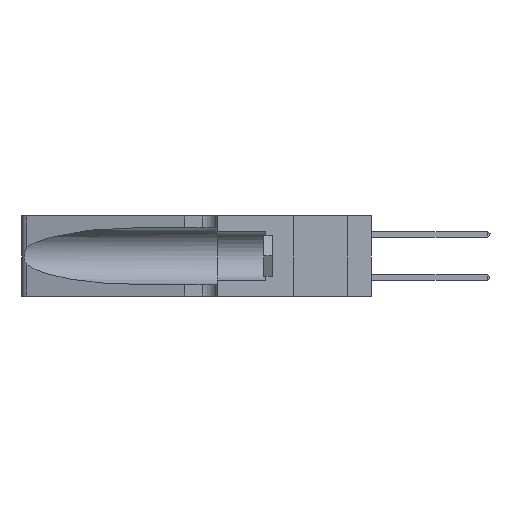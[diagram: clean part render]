
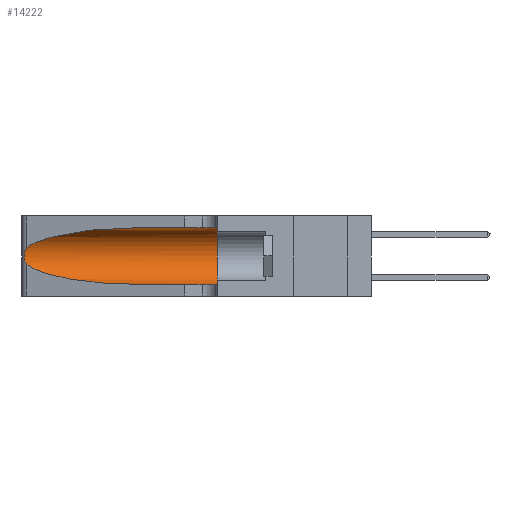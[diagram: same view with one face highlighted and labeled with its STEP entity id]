
A CAD part, left-side view. The second image highlights one B-rep face of the part: STEP entity #14222.
In plain terms, the highlighted cylindrical face has radius 3.308 mm (diameter 6.617 mm), a partial arc.
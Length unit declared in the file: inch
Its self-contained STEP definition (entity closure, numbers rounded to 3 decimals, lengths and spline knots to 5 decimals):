
#1465 = ORIENTED_EDGE ( 'NONE', *, *, #5780, .T. ) ;
#3020 = CARTESIAN_POINT ( 'NONE',  ( 0.26018, 1.23835, 0.19895 ) ) ;
#3657 = CARTESIAN_POINT ( 'NONE',  ( 0.1305, 1.61858, 0.31525 ) ) ;
#4451 = ORIENTED_EDGE ( 'NONE', *, *, #7092, .F. ) ;
#5444 = VERTEX_POINT ( 'NONE', #39725 ) ;
#5780 = EDGE_CURVE ( 'NONE', #19004, #22588, #9707, .T. ) ;
#6169 = CARTESIAN_POINT ( 'NONE',  ( 0.26075, 1.23896, 0.178 ) ) ;
#6817 = DIRECTION ( 'NONE',  ( 0., -1., 0. ) ) ;
#7053 = CARTESIAN_POINT ( 'NONE',  ( 0.18966, 0.96281, 0.31525 ) ) ;
#7092 = EDGE_CURVE ( 'NONE', #5444, #11283, #16973, .T. ) ;
#7350 = CIRCLE ( 'NONE', #20508, 0.13025 ) ;
#7450 =( BOUNDED_CURVE ( )  B_SPLINE_CURVE ( 3, ( #22784, #7053, #32101, #13344 ),
 .UNSPECIFIED., .F., .T. ) 
 B_SPLINE_CURVE_WITH_KNOTS ( ( 4, 4 ),
 ( 1.5708, 2.84003 ),
 .UNSPECIFIED. ) 
 CURVE ( )  GEOMETRIC_REPRESENTATION_ITEM ( )  RATIONAL_B_SPLINE_CURVE ( ( 1., 0.87, 0.87, 1. ) ) 
 REPRESENTATION_ITEM ( '' )  );
#9331 = CARTESIAN_POINT ( 'NONE',  ( 0.25856, 1.23593, 0.16098 ) ) ;
#9366 = CARTESIAN_POINT ( 'NONE',  ( 0.1305, 0.35, 0.185 ) ) ;
#9707 = LINE ( 'NONE', #35671, #24515 ) ;
#10033 = DIRECTION ( 'NONE',  ( 0., -1., 0. ) ) ;
#11283 = VERTEX_POINT ( 'NONE', #18541 ) ;
#11293 = EDGE_CURVE ( 'NONE', #24892, #19004, #29318, .T. ) ;
#12170 = CARTESIAN_POINT ( 'NONE',  ( 0.2373, 1.15595, 0.08982 ) ) ;
#12479 = CARTESIAN_POINT ( 'NONE',  ( 0.25639, 1.23186, 0.15144 ) ) ;
#12515 = DIRECTION ( 'NONE',  ( 0., 0., 1. ) ) ;
#13344 = CARTESIAN_POINT ( 'NONE',  ( 0.25487, 1.22718, 0.22369 ) ) ;
#14222 = ADVANCED_FACE ( 'NONE', ( #39668 ), #14785, .F. ) ;
#14785 = CYLINDRICAL_SURFACE ( 'NONE', #23349, 0.13025 ) ;
#15217 = ORIENTED_EDGE ( 'NONE', *, *, #11293, .T. ) ;
#15643 = CARTESIAN_POINT ( 'NONE',  ( 0.25487, 1.22718, 0.14631 ) ) ;
#16217 = DIRECTION ( 'NONE',  ( 0., 0., -1. ) ) ;
#16973 = LINE ( 'NONE', #3657, #32594 ) ;
#17548 = EDGE_CURVE ( 'NONE', #11283, #22588, #7350, .T. ) ;
#17898 = CARTESIAN_POINT ( 'NONE',  ( 0.25487, 1.22718, 0.22369 ) ) ;
#18541 = CARTESIAN_POINT ( 'NONE',  ( 0.1305, 0.35, 0.31525 ) ) ;
#18718 = CARTESIAN_POINT ( 'NONE',  ( 0.25639, 1.23184, 0.21858 ) ) ;
#19004 = VERTEX_POINT ( 'NONE', #30105 ) ;
#19424 = CARTESIAN_POINT ( 'NONE',  ( 0.1305, 1.61858, 0.185 ) ) ;
#19872 = EDGE_LOOP ( 'NONE', ( #25111, #20700, #15217, #1465, #34767, #4451 ) ) ;
#20417 = VERTEX_POINT ( 'NONE', #17898 ) ;
#20508 = AXIS2_PLACEMENT_3D ( 'NONE', #9366, #31275, #12515 ) ;
#20700 = ORIENTED_EDGE ( 'NONE', *, *, #29916, .T. ) ;
#21927 = CARTESIAN_POINT ( 'NONE',  ( 0.25854, 1.2359, 0.20912 ) ) ;
#22588 = VERTEX_POINT ( 'NONE', #33919 ) ;
#22784 = CARTESIAN_POINT ( 'NONE',  ( 0.1305, 0.72297, 0.31525 ) ) ;
#23349 = AXIS2_PLACEMENT_3D ( 'NONE', #19424, #10033, #16217 ) ;
#23379 = DIRECTION ( 'NONE',  ( 0., -1., 0. ) ) ;
#23480 = EDGE_CURVE ( 'NONE', #5444, #20417, #7450, .T. ) ;
#24515 = VECTOR ( 'NONE', #23379, 39.37008 ) ;
#24892 = VERTEX_POINT ( 'NONE', #28126 ) ;
#25055 = CARTESIAN_POINT ( 'NONE',  ( 0.26075, 1.23896, 0.19203 ) ) ;
#25111 = ORIENTED_EDGE ( 'NONE', *, *, #23480, .T. ) ;
#26378 = B_SPLINE_CURVE_WITH_KNOTS ( 'NONE', 3,
 ( #34199, #37338, #18718, #40406, #21927, #3020, #25055, #6169, #28136, #9331, #31241, #12479, #34334, #15643 ),
 .UNSPECIFIED., .F., .F.,
 ( 4, 2, 2, 2, 2, 2, 4 ),
 ( 0., 0.00027, 0.00053, 0.00107, 0.0016, 0.00187, 0.00214 ),
 .UNSPECIFIED. ) ;
#27959 = CARTESIAN_POINT ( 'NONE',  ( 0.25487, 1.22718, 0.14631 ) ) ;
#28126 = CARTESIAN_POINT ( 'NONE',  ( 0.25487, 1.22718, 0.14631 ) ) ;
#28136 = CARTESIAN_POINT ( 'NONE',  ( 0.26017, 1.23833, 0.17102 ) ) ;
#29318 =( BOUNDED_CURVE ( )  B_SPLINE_CURVE ( 3, ( #27959, #12170, #40232, #31062 ),
 .UNSPECIFIED., .F., .F. ) 
 B_SPLINE_CURVE_WITH_KNOTS ( ( 4, 4 ),
 ( 3.44316, 4.71239 ),
 .UNSPECIFIED. ) 
 CURVE ( )  GEOMETRIC_REPRESENTATION_ITEM ( )  RATIONAL_B_SPLINE_CURVE ( ( 1., 0.87, 0.87, 1. ) ) 
 REPRESENTATION_ITEM ( '' )  );
#29916 = EDGE_CURVE ( 'NONE', #20417, #24892, #26378, .T. ) ;
#30105 = CARTESIAN_POINT ( 'NONE',  ( 0.1305, 0.72297, 0.05475 ) ) ;
#31062 = CARTESIAN_POINT ( 'NONE',  ( 0.1305, 0.72297, 0.05475 ) ) ;
#31241 = CARTESIAN_POINT ( 'NONE',  ( 0.25789, 1.23486, 0.15765 ) ) ;
#31275 = DIRECTION ( 'NONE',  ( 0., 1., 0. ) ) ;
#32101 = CARTESIAN_POINT ( 'NONE',  ( 0.2373, 1.15595, 0.28018 ) ) ;
#32594 = VECTOR ( 'NONE', #6817, 39.37008 ) ;
#33919 = CARTESIAN_POINT ( 'NONE',  ( 0.1305, 0.35, 0.05475 ) ) ;
#34199 = CARTESIAN_POINT ( 'NONE',  ( 0.25487, 1.22718, 0.22369 ) ) ;
#34334 = CARTESIAN_POINT ( 'NONE',  ( 0.25555, 1.22993, 0.14849 ) ) ;
#34767 = ORIENTED_EDGE ( 'NONE', *, *, #17548, .F. ) ;
#35671 = CARTESIAN_POINT ( 'NONE',  ( 0.1305, 1.61858, 0.05475 ) ) ;
#37338 = CARTESIAN_POINT ( 'NONE',  ( 0.25555, 1.22994, 0.2215 ) ) ;
#39668 = FACE_OUTER_BOUND ( 'NONE', #19872, .T. ) ;
#39725 = CARTESIAN_POINT ( 'NONE',  ( 0.1305, 0.72297, 0.31525 ) ) ;
#40232 = CARTESIAN_POINT ( 'NONE',  ( 0.18966, 0.96281, 0.05475 ) ) ;
#40406 = CARTESIAN_POINT ( 'NONE',  ( 0.25787, 1.23484, 0.2124 ) ) ;
